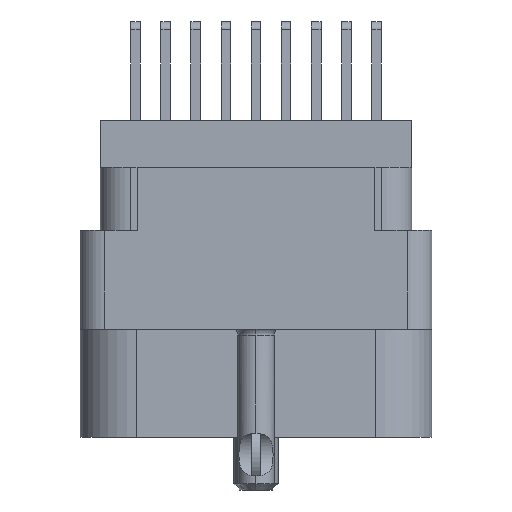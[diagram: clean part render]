
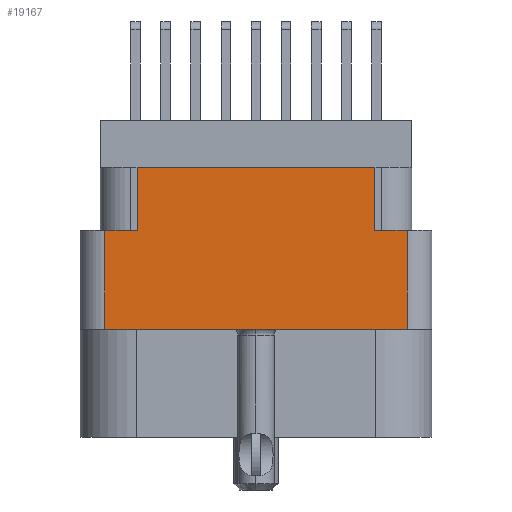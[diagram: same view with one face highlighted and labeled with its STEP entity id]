
A CAD part, left-side view. The second image highlights one B-rep face of the part: STEP entity #19167.
In plain terms, the highlighted planar face has unit normal (-1, 0, 0).
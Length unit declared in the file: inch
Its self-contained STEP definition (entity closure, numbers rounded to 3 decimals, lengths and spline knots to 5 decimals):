
#505 = VERTEX_POINT ( 'NONE', #43235 ) ;
#1816 = CARTESIAN_POINT ( 'NONE',  ( -1.2955, 0.376, -0.789 ) ) ;
#2249 = ORIENTED_EDGE ( 'NONE', *, *, #17290, .T. ) ;
#4785 = LINE ( 'NONE', #41049, #46527 ) ;
#4792 = VERTEX_POINT ( 'NONE', #47687 ) ;
#4913 = LINE ( 'NONE', #41172, #49854 ) ;
#5575 = EDGE_CURVE ( 'NONE', #48627, #505, #19047, .T. ) ;
#6205 = LINE ( 'NONE', #19287, #17399 ) ;
#6274 = DIRECTION ( 'NONE',  ( 0., 0., -1. ) ) ;
#7769 = ORIENTED_EDGE ( 'NONE', *, *, #15427, .F. ) ;
#9210 = EDGE_CURVE ( 'NONE', #10574, #50558, #42872, .T. ) ;
#10265 = PLANE ( 'NONE',  #10576 ) ;
#10404 = EDGE_LOOP ( 'NONE', ( #32013, #57286, #40941, #2249, #7769, #18953, #24244, #29018 ) ) ;
#10574 = VERTEX_POINT ( 'NONE', #58741 ) ;
#10576 = AXIS2_PLACEMENT_3D ( 'NONE', #42944, #32882, #28705 ) ;
#13898 = DIRECTION ( 'NONE',  ( 0., 0., 1. ) ) ;
#15286 = VERTEX_POINT ( 'NONE', #58482 ) ;
#15427 = EDGE_CURVE ( 'NONE', #27761, #28737, #48689, .T. ) ;
#15443 = EDGE_CURVE ( 'NONE', #27761, #15286, #57898, .T. ) ;
#15886 = EDGE_CURVE ( 'NONE', #4792, #505, #46986, .T. ) ;
#17290 = EDGE_CURVE ( 'NONE', #48627, #28737, #4785, .T. ) ;
#17399 = VECTOR ( 'NONE', #51379, 39.37008 ) ;
#18953 = ORIENTED_EDGE ( 'NONE', *, *, #15443, .T. ) ;
#19047 = LINE ( 'NONE', #56477, #34703 ) ;
#19167 = ADVANCED_FACE ( 'NONE', ( #46540 ), #10265, .T. ) ;
#19287 = CARTESIAN_POINT ( 'NONE',  ( -1.2955, 0.438, -0.117 ) ) ;
#19419 = VECTOR ( 'NONE', #13898, 39.37008 ) ;
#20421 = VECTOR ( 'NONE', #6274, 39.37008 ) ;
#20456 = EDGE_CURVE ( 'NONE', #50558, #15286, #6205, .T. ) ;
#22467 = EDGE_CURVE ( 'NONE', #4792, #10574, #4913, .T. ) ;
#24244 = ORIENTED_EDGE ( 'NONE', *, *, #20456, .F. ) ;
#27761 = VERTEX_POINT ( 'NONE', #40694 ) ;
#28705 = DIRECTION ( 'NONE',  ( 0., 0., 1. ) ) ;
#28737 = VERTEX_POINT ( 'NONE', #31278 ) ;
#29018 = ORIENTED_EDGE ( 'NONE', *, *, #9210, .F. ) ;
#31278 = CARTESIAN_POINT ( 'NONE',  ( -1.2955, -0.376, -0.274 ) ) ;
#31743 = CARTESIAN_POINT ( 'NONE',  ( -1.2955, 0., -0.274 ) ) ;
#32013 = ORIENTED_EDGE ( 'NONE', *, *, #22467, .F. ) ;
#32882 = DIRECTION ( 'NONE',  ( -1., 0., 0. ) ) ;
#34703 = VECTOR ( 'NONE', #52011, 39.37008 ) ;
#36606 = DIRECTION ( 'NONE',  ( 0., 0., 1. ) ) ;
#38031 = CARTESIAN_POINT ( 'NONE',  ( -1.2955, 0.296, -0.117 ) ) ;
#40694 = CARTESIAN_POINT ( 'NONE',  ( -1.2955, -0.296, -0.274 ) ) ;
#40941 = ORIENTED_EDGE ( 'NONE', *, *, #5575, .F. ) ;
#41049 = CARTESIAN_POINT ( 'NONE',  ( -1.2955, -0.376, -0.789 ) ) ;
#41172 = CARTESIAN_POINT ( 'NONE',  ( -1.2955, 0., -0.274 ) ) ;
#42872 = LINE ( 'NONE', #55959, #56907 ) ;
#42944 = CARTESIAN_POINT ( 'NONE',  ( -1.2955, -0.438, -0.789 ) ) ;
#43235 = CARTESIAN_POINT ( 'NONE',  ( -1.2955, 0.376, -0.52 ) ) ;
#46527 = VECTOR ( 'NONE', #36606, 39.37008 ) ;
#46540 = FACE_OUTER_BOUND ( 'NONE', #10404, .T. ) ;
#46986 = LINE ( 'NONE', #1816, #20421 ) ;
#47031 = DIRECTION ( 'NONE',  ( 0., 0., 1. ) ) ;
#47687 = CARTESIAN_POINT ( 'NONE',  ( -1.2955, 0.376, -0.274 ) ) ;
#48627 = VERTEX_POINT ( 'NONE', #49316 ) ;
#48689 = LINE ( 'NONE', #31743, #48877 ) ;
#48877 = VECTOR ( 'NONE', #58775, 39.37008 ) ;
#49316 = CARTESIAN_POINT ( 'NONE',  ( -1.2955, -0.376, -0.52 ) ) ;
#49854 = VECTOR ( 'NONE', #50663, 39.37008 ) ;
#50558 = VERTEX_POINT ( 'NONE', #38031 ) ;
#50663 = DIRECTION ( 'NONE',  ( 0., -1., 0. ) ) ;
#51379 = DIRECTION ( 'NONE',  ( 0., -1., 0. ) ) ;
#52011 = DIRECTION ( 'NONE',  ( 0., 1., 0. ) ) ;
#53446 = CARTESIAN_POINT ( 'NONE',  ( -1.2955, -0.296, -0.274 ) ) ;
#55959 = CARTESIAN_POINT ( 'NONE',  ( -1.2955, 0.296, -0.274 ) ) ;
#56477 = CARTESIAN_POINT ( 'NONE',  ( -1.2955, 0., -0.52 ) ) ;
#56907 = VECTOR ( 'NONE', #47031, 39.37008 ) ;
#57286 = ORIENTED_EDGE ( 'NONE', *, *, #15886, .T. ) ;
#57898 = LINE ( 'NONE', #53446, #19419 ) ;
#58482 = CARTESIAN_POINT ( 'NONE',  ( -1.2955, -0.296, -0.117 ) ) ;
#58741 = CARTESIAN_POINT ( 'NONE',  ( -1.2955, 0.296, -0.274 ) ) ;
#58775 = DIRECTION ( 'NONE',  ( 0., -1., 0. ) ) ;
